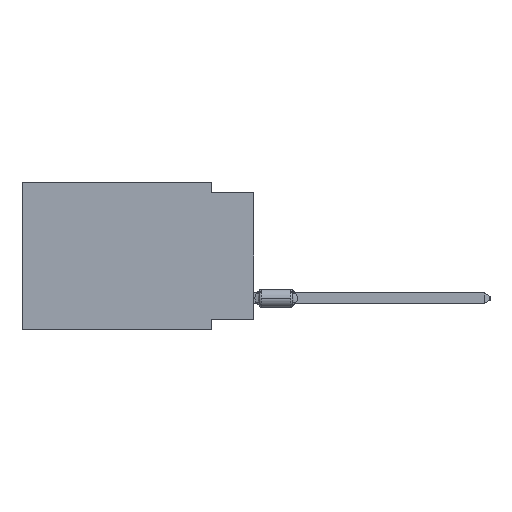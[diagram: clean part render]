
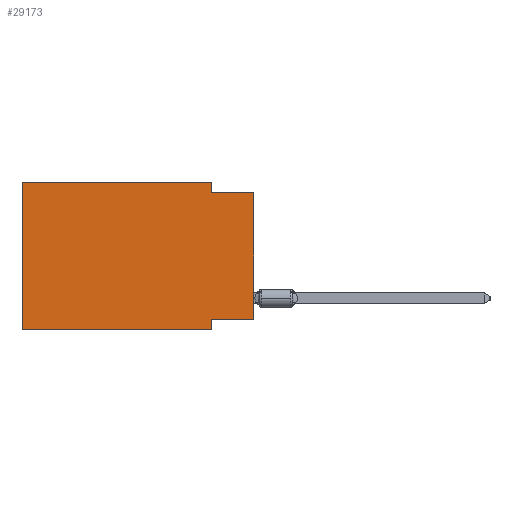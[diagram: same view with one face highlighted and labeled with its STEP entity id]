
A CAD part, left-side view. The second image highlights one B-rep face of the part: STEP entity #29173.
In plain terms, the highlighted planar face has unit normal (-1, 0, 0).
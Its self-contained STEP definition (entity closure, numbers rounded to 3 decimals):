
#159 = CARTESIAN_POINT ( 'NONE',  ( 0., 13.97, -8.89 ) ) ;
#216 = LINE ( 'NONE', #5562, #27524 ) ;
#248 = VERTEX_POINT ( 'NONE', #16566 ) ;
#332 = LINE ( 'NONE', #825, #28410 ) ;
#825 = CARTESIAN_POINT ( 'NONE',  ( 0., 0., -8.255 ) ) ;
#1572 = VECTOR ( 'NONE', #29768, 1000. ) ;
#2587 = EDGE_CURVE ( 'NONE', #29135, #10756, #216, .T. ) ;
#2626 = EDGE_CURVE ( 'NONE', #3743, #10756, #24804, .T. ) ;
#3387 = CARTESIAN_POINT ( 'NONE',  ( 0., 0., -0.635 ) ) ;
#3622 = EDGE_CURVE ( 'NONE', #10608, #18458, #11203, .T. ) ;
#3743 = VERTEX_POINT ( 'NONE', #22181 ) ;
#4314 = CARTESIAN_POINT ( 'NONE',  ( 0., 2.54, -8.255 ) ) ;
#5562 = CARTESIAN_POINT ( 'NONE',  ( 0., 0., -0.635 ) ) ;
#5767 = ORIENTED_EDGE ( 'NONE', *, *, #2587, .F. ) ;
#6199 = CARTESIAN_POINT ( 'NONE',  ( 0., 2.54, 0. ) ) ;
#7967 = DIRECTION ( 'NONE',  ( 0., 0., 1. ) ) ;
#8656 = DIRECTION ( 'NONE',  ( 0., -1., 0. ) ) ;
#8929 = CARTESIAN_POINT ( 'NONE',  ( 0., 13.97, 0. ) ) ;
#9604 = DIRECTION ( 'NONE',  ( 0., 0., -1. ) ) ;
#10078 = DIRECTION ( 'NONE',  ( 1., 0., 0. ) ) ;
#10203 = DIRECTION ( 'NONE',  ( 0., 1., 0. ) ) ;
#10243 = PLANE ( 'NONE',  #19926 ) ;
#10397 = DIRECTION ( 'NONE',  ( 0., -1., 0. ) ) ;
#10556 = EDGE_LOOP ( 'NONE', ( #15457, #5767, #28377, #16850, #20164, #24831, #29187, #15813 ) ) ;
#10608 = VERTEX_POINT ( 'NONE', #159 ) ;
#10756 = VERTEX_POINT ( 'NONE', #3387 ) ;
#11060 = DIRECTION ( 'NONE',  ( 0., 0., -1. ) ) ;
#11203 = LINE ( 'NONE', #8929, #21436 ) ;
#12671 = FACE_OUTER_BOUND ( 'NONE', #10556, .T. ) ;
#12956 = CARTESIAN_POINT ( 'NONE',  ( 0., 13.97, -8.89 ) ) ;
#13517 = CARTESIAN_POINT ( 'NONE',  ( 0., 13.97, 0. ) ) ;
#14350 = EDGE_CURVE ( 'NONE', #28549, #248, #24423, .T. ) ;
#15457 = ORIENTED_EDGE ( 'NONE', *, *, #2626, .T. ) ;
#15565 = CARTESIAN_POINT ( 'NONE',  ( 0., 2.54, 0. ) ) ;
#15813 = ORIENTED_EDGE ( 'NONE', *, *, #26989, .F. ) ;
#16566 = CARTESIAN_POINT ( 'NONE',  ( 0., 2.54, -8.89 ) ) ;
#16850 = ORIENTED_EDGE ( 'NONE', *, *, #25103, .F. ) ;
#17617 = CARTESIAN_POINT ( 'NONE',  ( 0., 13.97, 0. ) ) ;
#17990 = LINE ( 'NONE', #12956, #1572 ) ;
#18458 = VERTEX_POINT ( 'NONE', #17617 ) ;
#19491 = CARTESIAN_POINT ( 'NONE',  ( 0., 2.54, -0.635 ) ) ;
#19926 = AXIS2_PLACEMENT_3D ( 'NONE', #21909, #10078, #9604 ) ;
#20110 = VECTOR ( 'NONE', #31876, 1000. ) ;
#20164 = ORIENTED_EDGE ( 'NONE', *, *, #3622, .F. ) ;
#20303 = VECTOR ( 'NONE', #7967, 1000. ) ;
#21236 = DIRECTION ( 'NONE',  ( 0., 0., 1. ) ) ;
#21436 = VECTOR ( 'NONE', #21236, 1000. ) ;
#21909 = CARTESIAN_POINT ( 'NONE',  ( 0., 13.97, 0. ) ) ;
#22181 = CARTESIAN_POINT ( 'NONE',  ( 0., 0., -8.255 ) ) ;
#23528 = LINE ( 'NONE', #13517, #26689 ) ;
#24423 = LINE ( 'NONE', #29912, #20110 ) ;
#24804 = LINE ( 'NONE', #30132, #20303 ) ;
#24831 = ORIENTED_EDGE ( 'NONE', *, *, #26970, .T. ) ;
#25103 = EDGE_CURVE ( 'NONE', #18458, #28158, #23528, .T. ) ;
#26253 = LINE ( 'NONE', #6199, #28988 ) ;
#26689 = VECTOR ( 'NONE', #8656, 1000. ) ;
#26970 = EDGE_CURVE ( 'NONE', #10608, #248, #17990, .T. ) ;
#26989 = EDGE_CURVE ( 'NONE', #3743, #28549, #332, .T. ) ;
#27524 = VECTOR ( 'NONE', #10397, 1000. ) ;
#27951 = EDGE_CURVE ( 'NONE', #28158, #29135, #26253, .T. ) ;
#28158 = VERTEX_POINT ( 'NONE', #15565 ) ;
#28377 = ORIENTED_EDGE ( 'NONE', *, *, #27951, .F. ) ;
#28410 = VECTOR ( 'NONE', #10203, 1000. ) ;
#28549 = VERTEX_POINT ( 'NONE', #4314 ) ;
#28988 = VECTOR ( 'NONE', #11060, 1000. ) ;
#29135 = VERTEX_POINT ( 'NONE', #19491 ) ;
#29173 = ADVANCED_FACE ( 'NONE', ( #12671 ), #10243, .F. ) ;
#29187 = ORIENTED_EDGE ( 'NONE', *, *, #14350, .F. ) ;
#29768 = DIRECTION ( 'NONE',  ( 0., -1., 0. ) ) ;
#29912 = CARTESIAN_POINT ( 'NONE',  ( 0., 2.54, -8.89 ) ) ;
#30132 = CARTESIAN_POINT ( 'NONE',  ( 0., 0., 0. ) ) ;
#31876 = DIRECTION ( 'NONE',  ( 0., 0., -1. ) ) ;
